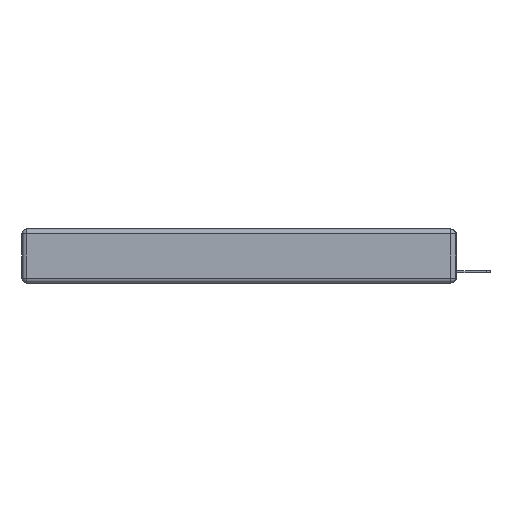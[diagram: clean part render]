
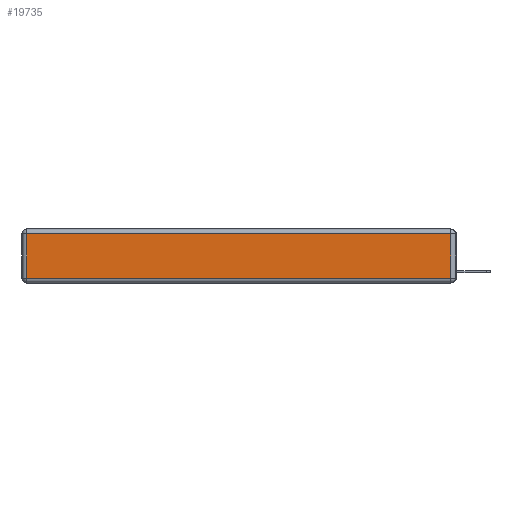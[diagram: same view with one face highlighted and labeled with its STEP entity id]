
A CAD part, left-side view. The second image highlights one B-rep face of the part: STEP entity #19735.
In plain terms, the highlighted planar face has unit normal (-1, 0, 0).
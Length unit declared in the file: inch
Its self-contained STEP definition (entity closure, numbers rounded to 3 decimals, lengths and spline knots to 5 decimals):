
#37 = EDGE_CURVE ( 'NONE', #24404, #8393, #9464, .T. ) ;
#541 = CARTESIAN_POINT ( 'NONE',  ( 0., 0., -0.313 ) ) ;
#963 = CARTESIAN_POINT ( 'NONE',  ( 0., 0., -0.343 ) ) ;
#1329 = LINE ( 'NONE', #3644, #26873 ) ;
#1461 = CARTESIAN_POINT ( 'NONE',  ( 0., 0.03, -0.313 ) ) ;
#3497 = LINE ( 'NONE', #12286, #7950 ) ;
#3644 = CARTESIAN_POINT ( 'NONE',  ( 0., 2.72, -0.343 ) ) ;
#7043 = DIRECTION ( 'NONE',  ( 0., -1., 0. ) ) ;
#7339 = LINE ( 'NONE', #541, #15670 ) ;
#7950 = VECTOR ( 'NONE', #10117, 39.37008 ) ;
#8393 = VERTEX_POINT ( 'NONE', #19862 ) ;
#9114 = CARTESIAN_POINT ( 'NONE',  ( 0., 2.72, -0.313 ) ) ;
#9182 = DIRECTION ( 'NONE',  ( 0., 1., 0. ) ) ;
#9464 = LINE ( 'NONE', #22582, #20134 ) ;
#10117 = DIRECTION ( 'NONE',  ( 0., 0., 1. ) ) ;
#10389 = ORIENTED_EDGE ( 'NONE', *, *, #17704, .T. ) ;
#10457 = VERTEX_POINT ( 'NONE', #9114 ) ;
#10663 = VERTEX_POINT ( 'NONE', #1461 ) ;
#12074 = DIRECTION ( 'NONE',  ( -1., 0., 0. ) ) ;
#12286 = CARTESIAN_POINT ( 'NONE',  ( 0., 0.03, -0.343 ) ) ;
#13965 = EDGE_LOOP ( 'NONE', ( #26242, #10389, #22026, #14813 ) ) ;
#14257 = EDGE_CURVE ( 'NONE', #10457, #10663, #7339, .T. ) ;
#14440 = CARTESIAN_POINT ( 'NONE',  ( 0., 0.03, -0.03 ) ) ;
#14813 = ORIENTED_EDGE ( 'NONE', *, *, #17650, .T. ) ;
#15670 = VECTOR ( 'NONE', #7043, 39.37008 ) ;
#16540 = FACE_OUTER_BOUND ( 'NONE', #13965, .T. ) ;
#17650 = EDGE_CURVE ( 'NONE', #8393, #10457, #1329, .T. ) ;
#17704 = EDGE_CURVE ( 'NONE', #10663, #24404, #3497, .T. ) ;
#18725 = DIRECTION ( 'NONE',  ( 0., 0., 1. ) ) ;
#19735 = ADVANCED_FACE ( 'NONE', ( #16540 ), #20740, .T. ) ;
#19862 = CARTESIAN_POINT ( 'NONE',  ( 0., 2.72, -0.03 ) ) ;
#20134 = VECTOR ( 'NONE', #9182, 39.37008 ) ;
#20740 = PLANE ( 'NONE',  #24588 ) ;
#22026 = ORIENTED_EDGE ( 'NONE', *, *, #37, .T. ) ;
#22582 = CARTESIAN_POINT ( 'NONE',  ( 0., 2.75, -0.03 ) ) ;
#24404 = VERTEX_POINT ( 'NONE', #14440 ) ;
#24588 = AXIS2_PLACEMENT_3D ( 'NONE', #963, #12074, #18725 ) ;
#25258 = DIRECTION ( 'NONE',  ( 0., 0., -1. ) ) ;
#26242 = ORIENTED_EDGE ( 'NONE', *, *, #14257, .T. ) ;
#26873 = VECTOR ( 'NONE', #25258, 39.37008 ) ;
